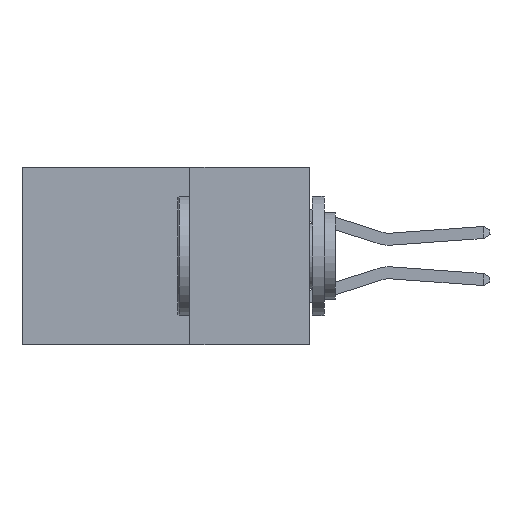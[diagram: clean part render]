
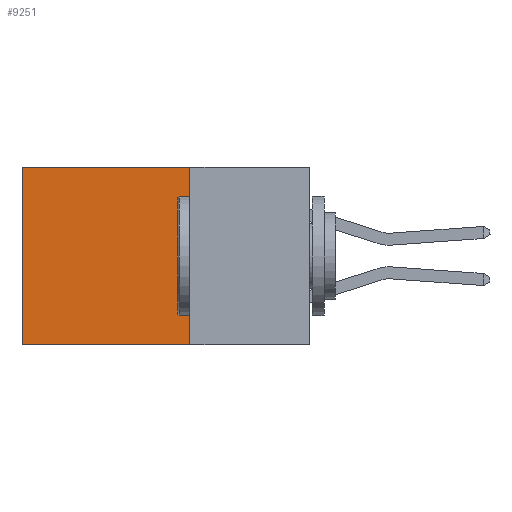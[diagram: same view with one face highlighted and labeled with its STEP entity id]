
A CAD part, left-side view. The second image highlights one B-rep face of the part: STEP entity #9251.
In plain terms, the highlighted planar face has unit normal (-1, 0, 0).
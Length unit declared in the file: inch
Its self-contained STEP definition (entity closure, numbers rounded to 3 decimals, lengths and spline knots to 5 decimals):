
#1644 = LINE ( 'NONE', #13545, #4654 ) ;
#2624 = CARTESIAN_POINT ( 'NONE',  ( 0.2615, 0.25, -0.37 ) ) ;
#3007 = CARTESIAN_POINT ( 'NONE',  ( 0.2615, 0.25, 0. ) ) ;
#3423 = LINE ( 'NONE', #12700, #11210 ) ;
#3723 = VERTEX_POINT ( 'NONE', #13573 ) ;
#4592 = DIRECTION ( 'NONE',  ( 0., 1., 0. ) ) ;
#4654 = VECTOR ( 'NONE', #12427, 39.37008 ) ;
#4700 = CARTESIAN_POINT ( 'NONE',  ( 0.2615, 0.25, -0.37 ) ) ;
#4780 = VECTOR ( 'NONE', #4592, 39.37008 ) ;
#4828 = VERTEX_POINT ( 'NONE', #4700 ) ;
#5335 = AXIS2_PLACEMENT_3D ( 'NONE', #14586, #8222, #9599 ) ;
#5556 = PLANE ( 'NONE',  #5335 ) ;
#5795 = ORIENTED_EDGE ( 'NONE', *, *, #16976, .T. ) ;
#6983 = CARTESIAN_POINT ( 'NONE',  ( 0.2615, 0.6, 0. ) ) ;
#7009 = FACE_OUTER_BOUND ( 'NONE', #9784, .T. ) ;
#7523 = VERTEX_POINT ( 'NONE', #6983 ) ;
#7984 = ORIENTED_EDGE ( 'NONE', *, *, #15312, .F. ) ;
#8024 = EDGE_CURVE ( 'NONE', #9676, #7523, #16342, .T. ) ;
#8222 = DIRECTION ( 'NONE',  ( 1., 0., 0. ) ) ;
#9103 = DIRECTION ( 'NONE',  ( 0., 0., -1. ) ) ;
#9251 = ADVANCED_FACE ( 'NONE', ( #7009 ), #5556, .F. ) ;
#9599 = DIRECTION ( 'NONE',  ( 0., 0., -1. ) ) ;
#9676 = VERTEX_POINT ( 'NONE', #14405 ) ;
#9784 = EDGE_LOOP ( 'NONE', ( #5795, #7984, #13519, #15829 ) ) ;
#11210 = VECTOR ( 'NONE', #15540, 39.37008 ) ;
#12427 = DIRECTION ( 'NONE',  ( 0., 0., -1. ) ) ;
#12700 = CARTESIAN_POINT ( 'NONE',  ( 0.2615, 0.25, -0.37 ) ) ;
#12830 = VECTOR ( 'NONE', #9103, 39.37008 ) ;
#13207 = LINE ( 'NONE', #2624, #12830 ) ;
#13519 = ORIENTED_EDGE ( 'NONE', *, *, #15380, .F. ) ;
#13545 = CARTESIAN_POINT ( 'NONE',  ( 0.2615, 0.6, -0.37 ) ) ;
#13573 = CARTESIAN_POINT ( 'NONE',  ( 0.2615, 0.6, -0.37 ) ) ;
#14405 = CARTESIAN_POINT ( 'NONE',  ( 0.2615, 0.25, 0. ) ) ;
#14586 = CARTESIAN_POINT ( 'NONE',  ( 0.2615, 0.25, -0.37 ) ) ;
#15312 = EDGE_CURVE ( 'NONE', #4828, #3723, #3423, .T. ) ;
#15380 = EDGE_CURVE ( 'NONE', #9676, #4828, #13207, .T. ) ;
#15540 = DIRECTION ( 'NONE',  ( 0., 1., 0. ) ) ;
#15829 = ORIENTED_EDGE ( 'NONE', *, *, #8024, .T. ) ;
#16342 = LINE ( 'NONE', #3007, #4780 ) ;
#16976 = EDGE_CURVE ( 'NONE', #7523, #3723, #1644, .T. ) ;
